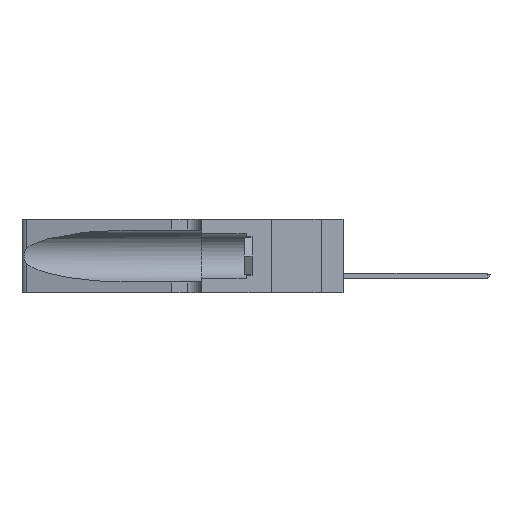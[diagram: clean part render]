
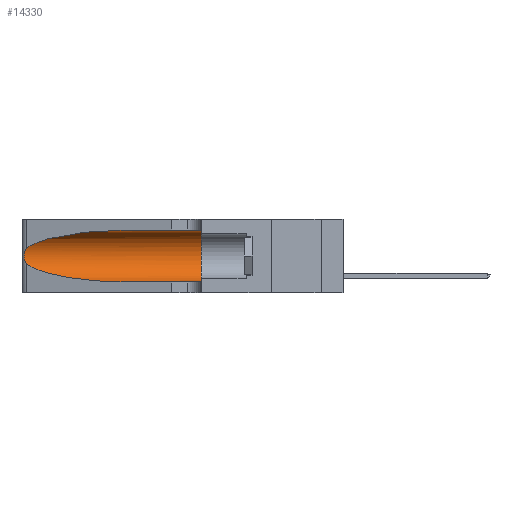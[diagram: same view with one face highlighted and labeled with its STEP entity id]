
A CAD part, left-side view. The second image highlights one B-rep face of the part: STEP entity #14330.
In plain terms, the highlighted cylindrical face has radius 3.308 mm (diameter 6.617 mm), a partial arc.
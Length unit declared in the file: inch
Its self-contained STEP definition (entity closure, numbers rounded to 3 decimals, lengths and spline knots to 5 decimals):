
#82 = ORIENTED_EDGE ( 'NONE', *, *, #22674, .F. ) ;
#150 = CARTESIAN_POINT ( 'NONE',  ( 0.1305, 1.61858, 0.05475 ) ) ;
#286 = CARTESIAN_POINT ( 'NONE',  ( 0.25487, 1.22718, 0.14631 ) ) ;
#389 = CARTESIAN_POINT ( 'NONE',  ( 0.26075, 1.23896, 0.178 ) ) ;
#745 = DIRECTION ( 'NONE',  ( 0., -1., 0. ) ) ;
#1234 = EDGE_CURVE ( 'NONE', #20452, #9120, #3530, .T. ) ;
#1955 = ORIENTED_EDGE ( 'NONE', *, *, #18347, .F. ) ;
#3530 =( BOUNDED_CURVE ( )  B_SPLINE_CURVE ( 3, ( #4934, #21126, #13874, #7439 ),
 .UNSPECIFIED., .F., .F. ) 
 B_SPLINE_CURVE_WITH_KNOTS ( ( 4, 4 ),
 ( 1.5708, 2.84003 ),
 .UNSPECIFIED. ) 
 CURVE ( )  GEOMETRIC_REPRESENTATION_ITEM ( )  RATIONAL_B_SPLINE_CURVE ( ( 1., 0.87, 0.87, 1. ) ) 
 REPRESENTATION_ITEM ( '' )  );
#3991 = CARTESIAN_POINT ( 'NONE',  ( 0.1305, 0.35, 0.31525 ) ) ;
#4670 = ORIENTED_EDGE ( 'NONE', *, *, #22242, .T. ) ;
#4934 = CARTESIAN_POINT ( 'NONE',  ( 0.1305, 0.72297, 0.31525 ) ) ;
#4940 = CARTESIAN_POINT ( 'NONE',  ( 0.25487, 1.22718, 0.22369 ) ) ;
#5125 = DIRECTION ( 'NONE',  ( 0., 0., -1. ) ) ;
#5232 = CARTESIAN_POINT ( 'NONE',  ( 0.25856, 1.23593, 0.16098 ) ) ;
#5384 = LINE ( 'NONE', #24727, #10114 ) ;
#7214 = CARTESIAN_POINT ( 'NONE',  ( 0.1305, 0.72297, 0.31525 ) ) ;
#7439 = CARTESIAN_POINT ( 'NONE',  ( 0.25487, 1.22718, 0.22369 ) ) ;
#7700 = CARTESIAN_POINT ( 'NONE',  ( 0.1305, 0.35, 0.185 ) ) ;
#8981 = ORIENTED_EDGE ( 'NONE', *, *, #11238, .T. ) ;
#9120 = VERTEX_POINT ( 'NONE', #23038 ) ;
#9320 = AXIS2_PLACEMENT_3D ( 'NONE', #7700, #15017, #17146 ) ;
#9606 = DIRECTION ( 'NONE',  ( 0., -1., 0. ) ) ;
#9845 = VERTEX_POINT ( 'NONE', #18770 ) ;
#10114 = VECTOR ( 'NONE', #22692, 39.37008 ) ;
#10480 = CYLINDRICAL_SURFACE ( 'NONE', #17695, 0.13025 ) ;
#11167 = B_SPLINE_CURVE_WITH_KNOTS ( 'NONE', 3,
 ( #4940, #16391, #21135, #18721, #11858, #28125, #18823, #389, #16689, #5232, #28021, #14188, #25590, #286 ),
 .UNSPECIFIED., .F., .F.,
 ( 4, 2, 2, 2, 2, 2, 4 ),
 ( 0., 0.00027, 0.00053, 0.00107, 0.0016, 0.00187, 0.00214 ),
 .UNSPECIFIED. ) ;
#11238 = EDGE_CURVE ( 'NONE', #9120, #16983, #11167, .T. ) ;
#11718 = CARTESIAN_POINT ( 'NONE',  ( 0.2373, 1.15595, 0.08982 ) ) ;
#11815 = EDGE_CURVE ( 'NONE', #20017, #9845, #29387, .T. ) ;
#11858 = CARTESIAN_POINT ( 'NONE',  ( 0.25854, 1.2359, 0.20912 ) ) ;
#13017 = FACE_OUTER_BOUND ( 'NONE', #26447, .T. ) ;
#13874 = CARTESIAN_POINT ( 'NONE',  ( 0.2373, 1.15595, 0.28018 ) ) ;
#14188 = CARTESIAN_POINT ( 'NONE',  ( 0.25639, 1.23186, 0.15144 ) ) ;
#14330 = ADVANCED_FACE ( 'NONE', ( #13017 ), #10480, .F. ) ;
#15017 = DIRECTION ( 'NONE',  ( 0., 1., 0. ) ) ;
#15578 = CARTESIAN_POINT ( 'NONE',  ( 0.25487, 1.22718, 0.14631 ) ) ;
#16303 = CARTESIAN_POINT ( 'NONE',  ( 0.1305, 0.72297, 0.05475 ) ) ;
#16391 = CARTESIAN_POINT ( 'NONE',  ( 0.25555, 1.22994, 0.2215 ) ) ;
#16689 = CARTESIAN_POINT ( 'NONE',  ( 0.26017, 1.23833, 0.17102 ) ) ;
#16983 = VERTEX_POINT ( 'NONE', #15578 ) ;
#17146 = DIRECTION ( 'NONE',  ( 0., 0., 1. ) ) ;
#17695 = AXIS2_PLACEMENT_3D ( 'NONE', #25872, #9606, #5125 ) ;
#18347 = EDGE_CURVE ( 'NONE', #25456, #9845, #27989, .T. ) ;
#18721 = CARTESIAN_POINT ( 'NONE',  ( 0.25787, 1.23484, 0.2124 ) ) ;
#18770 = CARTESIAN_POINT ( 'NONE',  ( 0.1305, 0.35, 0.05475 ) ) ;
#18781 = CARTESIAN_POINT ( 'NONE',  ( 0.1305, 0.72297, 0.05475 ) ) ;
#18823 = CARTESIAN_POINT ( 'NONE',  ( 0.26075, 1.23896, 0.19203 ) ) ;
#20017 = VERTEX_POINT ( 'NONE', #16303 ) ;
#20452 = VERTEX_POINT ( 'NONE', #7214 ) ;
#21126 = CARTESIAN_POINT ( 'NONE',  ( 0.18966, 0.96281, 0.31525 ) ) ;
#21135 = CARTESIAN_POINT ( 'NONE',  ( 0.25639, 1.23184, 0.21858 ) ) ;
#21404 = VECTOR ( 'NONE', #745, 39.37008 ) ;
#22242 = EDGE_CURVE ( 'NONE', #16983, #20017, #25966, .T. ) ;
#22674 = EDGE_CURVE ( 'NONE', #20452, #25456, #5384, .T. ) ;
#22692 = DIRECTION ( 'NONE',  ( 0., -1., 0. ) ) ;
#23038 = CARTESIAN_POINT ( 'NONE',  ( 0.25487, 1.22718, 0.22369 ) ) ;
#23215 = CARTESIAN_POINT ( 'NONE',  ( 0.25487, 1.22718, 0.14631 ) ) ;
#24727 = CARTESIAN_POINT ( 'NONE',  ( 0.1305, 1.61858, 0.31525 ) ) ;
#25456 = VERTEX_POINT ( 'NONE', #3991 ) ;
#25590 = CARTESIAN_POINT ( 'NONE',  ( 0.25555, 1.22993, 0.14849 ) ) ;
#25872 = CARTESIAN_POINT ( 'NONE',  ( 0.1305, 1.61858, 0.185 ) ) ;
#25966 =( BOUNDED_CURVE ( )  B_SPLINE_CURVE ( 3, ( #23215, #11718, #27685, #18781 ),
 .UNSPECIFIED., .F., .F. ) 
 B_SPLINE_CURVE_WITH_KNOTS ( ( 4, 4 ),
 ( 3.44316, 4.71239 ),
 .UNSPECIFIED. ) 
 CURVE ( )  GEOMETRIC_REPRESENTATION_ITEM ( )  RATIONAL_B_SPLINE_CURVE ( ( 1., 0.87, 0.87, 1. ) ) 
 REPRESENTATION_ITEM ( '' )  );
#26447 = EDGE_LOOP ( 'NONE', ( #29893, #8981, #4670, #28558, #1955, #82 ) ) ;
#27685 = CARTESIAN_POINT ( 'NONE',  ( 0.18966, 0.96281, 0.05475 ) ) ;
#27989 = CIRCLE ( 'NONE', #9320, 0.13025 ) ;
#28021 = CARTESIAN_POINT ( 'NONE',  ( 0.25789, 1.23486, 0.15765 ) ) ;
#28125 = CARTESIAN_POINT ( 'NONE',  ( 0.26018, 1.23835, 0.19895 ) ) ;
#28558 = ORIENTED_EDGE ( 'NONE', *, *, #11815, .T. ) ;
#29387 = LINE ( 'NONE', #150, #21404 ) ;
#29893 = ORIENTED_EDGE ( 'NONE', *, *, #1234, .T. ) ;
